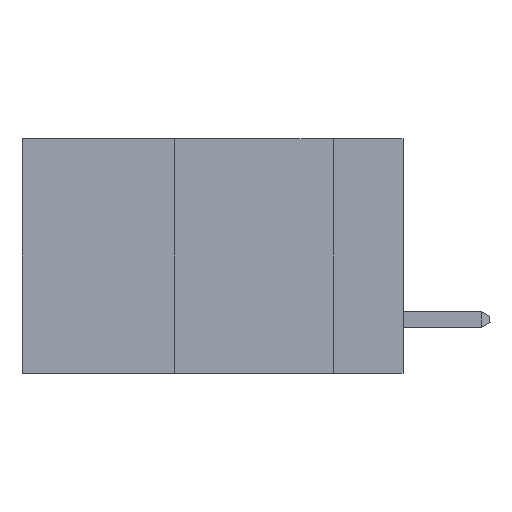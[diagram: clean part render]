
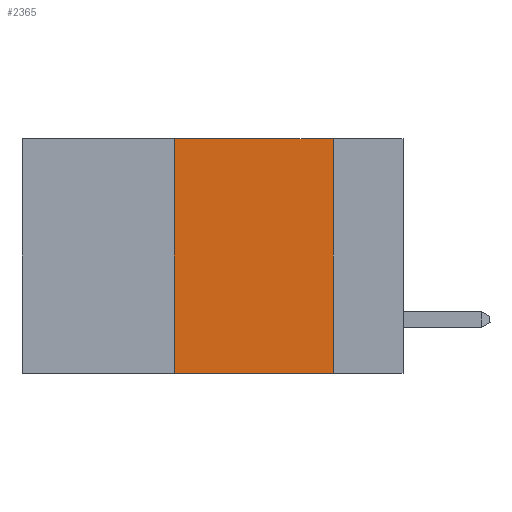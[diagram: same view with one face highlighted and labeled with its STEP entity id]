
A CAD part, left-side view. The second image highlights one B-rep face of the part: STEP entity #2365.
In plain terms, the highlighted planar face has unit normal (-1, 0, 0).
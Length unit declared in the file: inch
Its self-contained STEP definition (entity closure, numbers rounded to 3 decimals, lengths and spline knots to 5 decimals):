
#475 = CARTESIAN_POINT ( 'NONE',  ( 0., 0.36, 0. ) ) ;
#1466 = EDGE_CURVE ( 'NONE', #17878, #22408, #21557, .T. ) ;
#2365 = ADVANCED_FACE ( 'NONE', ( #28006 ), #8800, .F. ) ;
#5402 = EDGE_CURVE ( 'NONE', #17878, #24189, #25286, .T. ) ;
#7925 = CARTESIAN_POINT ( 'NONE',  ( 0., 0.11, 0. ) ) ;
#8189 = VECTOR ( 'NONE', #17569, 39.37008 ) ;
#8405 = EDGE_CURVE ( 'NONE', #8890, #22408, #15926, .T. ) ;
#8800 = PLANE ( 'NONE',  #23999 ) ;
#8890 = VERTEX_POINT ( 'NONE', #10840 ) ;
#9071 = EDGE_CURVE ( 'NONE', #24189, #8890, #26546, .T. ) ;
#10054 = CARTESIAN_POINT ( 'NONE',  ( 0., 0.11, -0.37 ) ) ;
#10840 = CARTESIAN_POINT ( 'NONE',  ( 0., 0.11, 0. ) ) ;
#11060 = DIRECTION ( 'NONE',  ( 0., 0., -1. ) ) ;
#12192 = VECTOR ( 'NONE', #25440, 39.37008 ) ;
#15478 = ORIENTED_EDGE ( 'NONE', *, *, #5402, .F. ) ;
#15926 = LINE ( 'NONE', #7925, #8189 ) ;
#17525 = VECTOR ( 'NONE', #28950, 39.37008 ) ;
#17569 = DIRECTION ( 'NONE',  ( 0., 0., -1. ) ) ;
#17738 = CARTESIAN_POINT ( 'NONE',  ( 0., 0.36, -0.37 ) ) ;
#17878 = VERTEX_POINT ( 'NONE', #17738 ) ;
#17881 = VECTOR ( 'NONE', #22967, 39.37008 ) ;
#18156 = CARTESIAN_POINT ( 'NONE',  ( 0., 0.6, 0. ) ) ;
#18240 = CARTESIAN_POINT ( 'NONE',  ( 0., 0.6, 0. ) ) ;
#18322 = EDGE_LOOP ( 'NONE', ( #29356, #21420, #15478, #22330 ) ) ;
#19714 = CARTESIAN_POINT ( 'NONE',  ( 0., 0.36, 0. ) ) ;
#21420 = ORIENTED_EDGE ( 'NONE', *, *, #9071, .F. ) ;
#21557 = LINE ( 'NONE', #30250, #17881 ) ;
#22330 = ORIENTED_EDGE ( 'NONE', *, *, #1466, .T. ) ;
#22408 = VERTEX_POINT ( 'NONE', #10054 ) ;
#22967 = DIRECTION ( 'NONE',  ( 0., -1., 0. ) ) ;
#23999 = AXIS2_PLACEMENT_3D ( 'NONE', #18156, #27412, #11060 ) ;
#24189 = VERTEX_POINT ( 'NONE', #475 ) ;
#25286 = LINE ( 'NONE', #19714, #17525 ) ;
#25440 = DIRECTION ( 'NONE',  ( 0., -1., 0. ) ) ;
#26546 = LINE ( 'NONE', #18240, #12192 ) ;
#27412 = DIRECTION ( 'NONE',  ( 1., 0., 0. ) ) ;
#28006 = FACE_OUTER_BOUND ( 'NONE', #18322, .T. ) ;
#28950 = DIRECTION ( 'NONE',  ( 0., 0., 1. ) ) ;
#29356 = ORIENTED_EDGE ( 'NONE', *, *, #8405, .F. ) ;
#30250 = CARTESIAN_POINT ( 'NONE',  ( 0., 0.6, -0.37 ) ) ;
